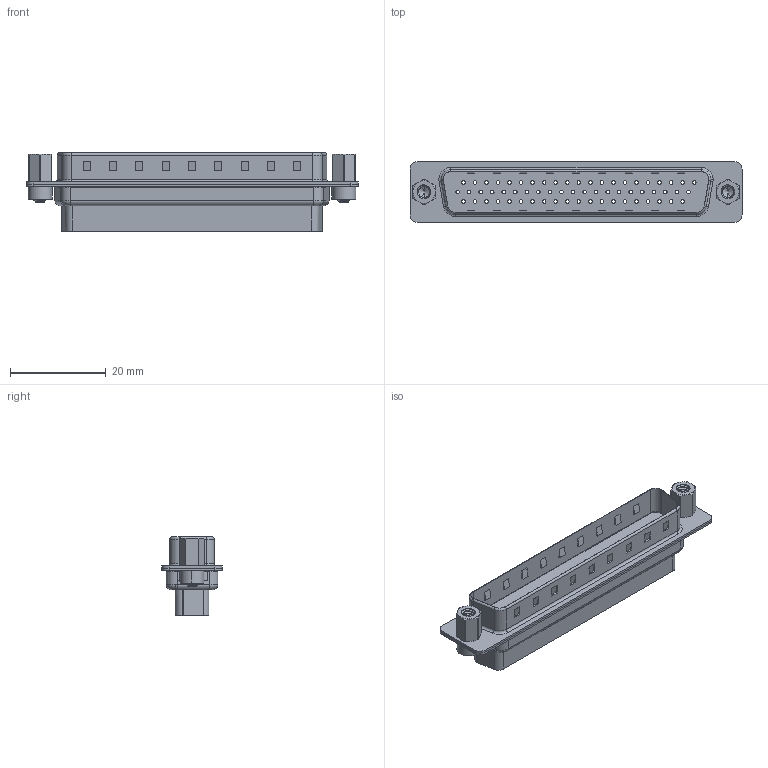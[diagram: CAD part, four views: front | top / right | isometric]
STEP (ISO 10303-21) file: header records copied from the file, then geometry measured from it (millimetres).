
FILE_DESCRIPTION (( 'STEP AP203' ), '1' );
FILE_NAME ('637-062-010-043.STEP', '2020-07-17T21:25:45', ( '' ), ( '' ), 'SwSTEP 2.0', 'SolidWorks 2020', '' );
FILE_SCHEMA (( 'CONFIG_CONTROL_DESIGN' ));
Length unit declared in the file: millimetre
Products named in the file (6): 637 Shell Front_62 Contacts; 637 4-40 Hex Standoff; 637 Housing_62 Contacts HP; 637 Shell Rear_62 Contacts; 637-062-010-043; 637 4-40 Threaded Rivet
Assembly tree (7 placements, depth 2):
  637-062-010-043
    637 Housing_62 Contacts HP
    637 Shell Front_62 Contacts
    637 Shell Rear_62 Contacts
    637 4-40 Threaded Rivet  x2
    637 4-40 Hex Standoff  x2
Bounding box: 69.4 x 12.6 x 16.4 mm (x, y, z)
Volume: 4370.6 mm3; surface area: 10276.7 mm2
Topology: 7 solids, 7 shells, 1034 faces, 2521 edges, 1636 vertices
Faces by surface type: cylinder 585, plane 349, torus 50, cone 32, bspline 18
Entity records: 32747 total; most frequent: CARTESIAN_POINT 9108, DIRECTION 5075, ORIENTED_EDGE 4528, EDGE_CURVE 2264, AXIS2_PLACEMENT_3D 2010, VERTEX_POINT 1471, EDGE_LOOP 1247, CIRCLE 1071
